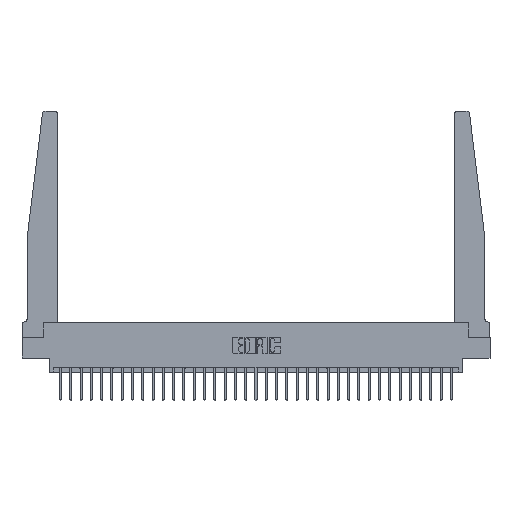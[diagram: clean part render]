
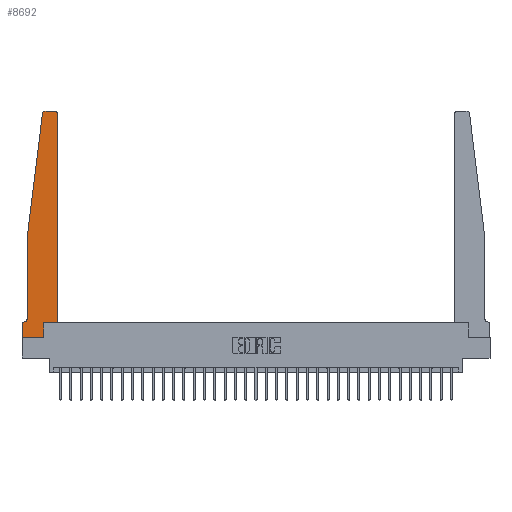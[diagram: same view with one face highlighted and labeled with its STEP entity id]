
A CAD part, top view. The second image highlights one B-rep face of the part: STEP entity #8692.
In plain terms, the highlighted planar face has unit normal (0, 0, 1).
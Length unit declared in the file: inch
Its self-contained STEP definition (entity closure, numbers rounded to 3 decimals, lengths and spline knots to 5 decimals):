
#50 = VERTEX_POINT ( 'NONE', #24066 ) ;
#606 = LINE ( 'NONE', #21841, #25242 ) ;
#636 = CARTESIAN_POINT ( 'NONE',  ( 0.2605, 0.18, 0.37 ) ) ;
#1083 = CARTESIAN_POINT ( 'NONE',  ( 0.425, 0.18, 0.37 ) ) ;
#1540 = FACE_OUTER_BOUND ( 'NONE', #26843, .T. ) ;
#2147 = DIRECTION ( 'NONE',  ( 1., 0., 0. ) ) ;
#2424 = VERTEX_POINT ( 'NONE', #9394 ) ;
#2498 = LINE ( 'NONE', #22197, #27054 ) ;
#2720 = VECTOR ( 'NONE', #15024, 39.37008 ) ;
#2837 = DIRECTION ( 'NONE',  ( 0., 0., -1. ) ) ;
#2967 = VERTEX_POINT ( 'NONE', #18457 ) ;
#3053 = CARTESIAN_POINT ( 'NONE',  ( 0.065, 1.25, 0.37 ) ) ;
#4462 = CIRCLE ( 'NONE', #26540, 0.03 ) ;
#4740 = VERTEX_POINT ( 'NONE', #636 ) ;
#4830 = CARTESIAN_POINT ( 'NONE',  ( 0.015, 0.1875, 0.37 ) ) ;
#5014 = EDGE_CURVE ( 'NONE', #4740, #28579, #27841, .T. ) ;
#5126 = VERTEX_POINT ( 'NONE', #30475 ) ;
#5332 = DIRECTION ( 'NONE',  ( 1., 0., 0. ) ) ;
#5371 = EDGE_CURVE ( 'NONE', #10846, #2424, #606, .T. ) ;
#5893 = ORIENTED_EDGE ( 'NONE', *, *, #27815, .T. ) ;
#6312 = VERTEX_POINT ( 'NONE', #4830 ) ;
#6893 = EDGE_CURVE ( 'NONE', #17223, #50, #10757, .T. ) ;
#7023 = VERTEX_POINT ( 'NONE', #21549 ) ;
#7075 = CARTESIAN_POINT ( 'NONE',  ( 0.27653, 2.75, 0.37 ) ) ;
#7705 = CARTESIAN_POINT ( 'NONE',  ( 0., 0.1875, 0.37 ) ) ;
#8577 = EDGE_CURVE ( 'NONE', #5126, #7023, #29808, .T. ) ;
#8692 = ADVANCED_FACE ( 'NONE', ( #1540 ), #17245, .T. ) ;
#9386 = CIRCLE ( 'NONE', #30743, 0.05 ) ;
#9394 = CARTESIAN_POINT ( 'NONE',  ( 0.065, 0.2375, 0.37 ) ) ;
#9713 = CARTESIAN_POINT ( 'NONE',  ( 0.395, 2.72, 0.37 ) ) ;
#10110 = CARTESIAN_POINT ( 'NONE',  ( 0.2605, 0.18, 0.37 ) ) ;
#10585 = DIRECTION ( 'NONE',  ( -0.122, -0.992, 0. ) ) ;
#10738 = DIRECTION ( 'NONE',  ( 0., 1., 0. ) ) ;
#10757 = LINE ( 'NONE', #28112, #16322 ) ;
#10846 = VERTEX_POINT ( 'NONE', #30740 ) ;
#11245 = ORIENTED_EDGE ( 'NONE', *, *, #5014, .T. ) ;
#11406 = DIRECTION ( 'NONE',  ( -1., 0., 0. ) ) ;
#12056 = DIRECTION ( 'NONE',  ( 1., 0., 0. ) ) ;
#12261 = EDGE_CURVE ( 'NONE', #2424, #6312, #9386, .T. ) ;
#12453 = DIRECTION ( 'NONE',  ( 0., 1., 0. ) ) ;
#13305 = VERTEX_POINT ( 'NONE', #7075 ) ;
#13323 = ORIENTED_EDGE ( 'NONE', *, *, #12261, .T. ) ;
#13700 = CARTESIAN_POINT ( 'NONE',  ( 0.425, 0.18, 0.37 ) ) ;
#13944 = AXIS2_PLACEMENT_3D ( 'NONE', #7705, #19618, #5332 ) ;
#15024 = DIRECTION ( 'NONE',  ( 0., -1., 0. ) ) ;
#15303 = VERTEX_POINT ( 'NONE', #19922 ) ;
#15599 = ORIENTED_EDGE ( 'NONE', *, *, #29414, .T. ) ;
#15668 = ORIENTED_EDGE ( 'NONE', *, *, #8577, .T. ) ;
#16084 = CARTESIAN_POINT ( 'NONE',  ( 0.25, 2.75, 0.37 ) ) ;
#16099 = DIRECTION ( 'NONE',  ( 1., 0., 0. ) ) ;
#16322 = VECTOR ( 'NONE', #21051, 39.37008 ) ;
#16416 = EDGE_CURVE ( 'NONE', #13305, #2967, #4462, .T. ) ;
#16529 = DIRECTION ( 'NONE',  ( 0., 0., 1. ) ) ;
#17199 = CARTESIAN_POINT ( 'NONE',  ( 0.015, 0.2375, 0.37 ) ) ;
#17223 = VERTEX_POINT ( 'NONE', #23783 ) ;
#17245 = PLANE ( 'NONE',  #13944 ) ;
#18457 = CARTESIAN_POINT ( 'NONE',  ( 0.24675, 2.72367, 0.37 ) ) ;
#18468 = LINE ( 'NONE', #10110, #25458 ) ;
#18604 = VECTOR ( 'NONE', #10738, 39.37008 ) ;
#19150 = ORIENTED_EDGE ( 'NONE', *, *, #22637, .T. ) ;
#19286 = VECTOR ( 'NONE', #10585, 39.37008 ) ;
#19454 = ORIENTED_EDGE ( 'NONE', *, *, #16416, .T. ) ;
#19574 = DIRECTION ( 'NONE',  ( -1., 0., 0. ) ) ;
#19618 = DIRECTION ( 'NONE',  ( 0., 0., 1. ) ) ;
#19922 = CARTESIAN_POINT ( 'NONE',  ( 0., 0.1875, 0.37 ) ) ;
#20854 = AXIS2_PLACEMENT_3D ( 'NONE', #9713, #26205, #12056 ) ;
#21051 = DIRECTION ( 'NONE',  ( 1., 0., 0. ) ) ;
#21075 = ORIENTED_EDGE ( 'NONE', *, *, #27031, .T. ) ;
#21380 = EDGE_CURVE ( 'NONE', #2967, #10846, #30095, .T. ) ;
#21549 = CARTESIAN_POINT ( 'NONE',  ( 0.395, 2.75, 0.37 ) ) ;
#21779 = LINE ( 'NONE', #26748, #2720 ) ;
#21841 = CARTESIAN_POINT ( 'NONE',  ( 0.065, 1.25, 0.37 ) ) ;
#21976 = ORIENTED_EDGE ( 'NONE', *, *, #6893, .T. ) ;
#22197 = CARTESIAN_POINT ( 'NONE',  ( 0.065, 0.1875, 0.37 ) ) ;
#22234 = VECTOR ( 'NONE', #11406, 39.37008 ) ;
#22637 = EDGE_CURVE ( 'NONE', #6312, #15303, #2498, .T. ) ;
#23670 = CARTESIAN_POINT ( 'NONE',  ( 0.425, 0.18, 0.37 ) ) ;
#23783 = CARTESIAN_POINT ( 'NONE',  ( 0., 0., 0.37 ) ) ;
#24066 = CARTESIAN_POINT ( 'NONE',  ( 0.2605, 0., 0.37 ) ) ;
#24839 = LINE ( 'NONE', #1083, #18604 ) ;
#25242 = VECTOR ( 'NONE', #28819, 39.37008 ) ;
#25458 = VECTOR ( 'NONE', #12453, 39.37008 ) ;
#26205 = DIRECTION ( 'NONE',  ( 0., 0., 1. ) ) ;
#26540 = AXIS2_PLACEMENT_3D ( 'NONE', #30601, #16529, #2147 ) ;
#26748 = CARTESIAN_POINT ( 'NONE',  ( 0., 0., 0.37 ) ) ;
#26843 = EDGE_LOOP ( 'NONE', ( #5893, #19454, #28492, #28985, #13323, #19150, #28749, #21976, #15599, #11245, #21075, #15668 ) ) ;
#26897 = DIRECTION ( 'NONE',  ( -1., 0., 0. ) ) ;
#27031 = EDGE_CURVE ( 'NONE', #28579, #5126, #24839, .T. ) ;
#27054 = VECTOR ( 'NONE', #26897, 39.37008 ) ;
#27094 = VECTOR ( 'NONE', #16099, 39.37008 ) ;
#27815 = EDGE_CURVE ( 'NONE', #7023, #13305, #28482, .T. ) ;
#27841 = LINE ( 'NONE', #13700, #27094 ) ;
#28112 = CARTESIAN_POINT ( 'NONE',  ( 0., 0., 0.37 ) ) ;
#28482 = LINE ( 'NONE', #16084, #22234 ) ;
#28492 = ORIENTED_EDGE ( 'NONE', *, *, #21380, .T. ) ;
#28579 = VERTEX_POINT ( 'NONE', #23670 ) ;
#28749 = ORIENTED_EDGE ( 'NONE', *, *, #30197, .T. ) ;
#28819 = DIRECTION ( 'NONE',  ( 0., -1., 0. ) ) ;
#28985 = ORIENTED_EDGE ( 'NONE', *, *, #5371, .T. ) ;
#29414 = EDGE_CURVE ( 'NONE', #50, #4740, #18468, .T. ) ;
#29808 = CIRCLE ( 'NONE', #20854, 0.03 ) ;
#30095 = LINE ( 'NONE', #3053, #19286 ) ;
#30197 = EDGE_CURVE ( 'NONE', #15303, #17223, #21779, .T. ) ;
#30475 = CARTESIAN_POINT ( 'NONE',  ( 0.425, 2.72, 0.37 ) ) ;
#30601 = CARTESIAN_POINT ( 'NONE',  ( 0.27653, 2.72, 0.37 ) ) ;
#30740 = CARTESIAN_POINT ( 'NONE',  ( 0.065, 1.25, 0.37 ) ) ;
#30743 = AXIS2_PLACEMENT_3D ( 'NONE', #17199, #2837, #19574 ) ;
